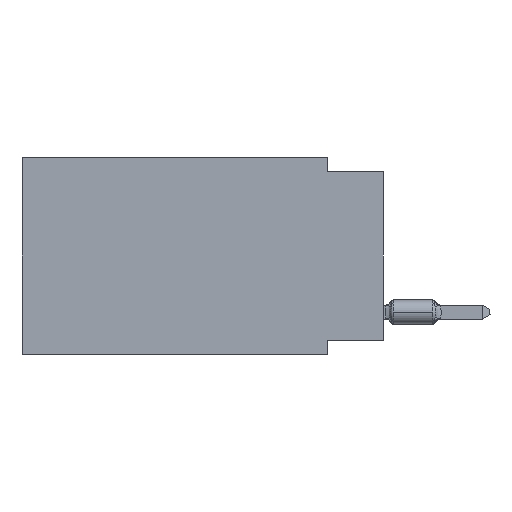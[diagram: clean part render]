
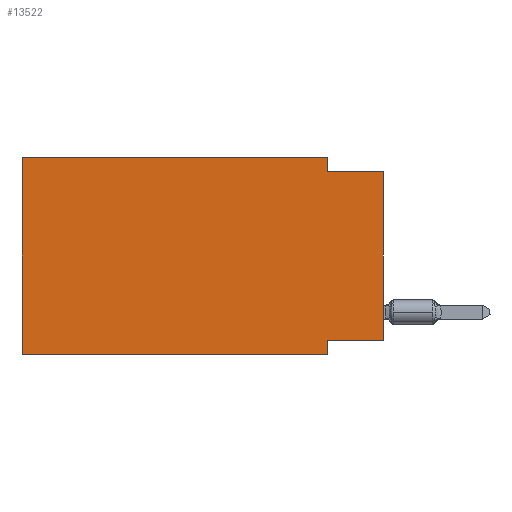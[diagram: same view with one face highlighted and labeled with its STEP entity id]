
A CAD part, left-side view. The second image highlights one B-rep face of the part: STEP entity #13522.
In plain terms, the highlighted planar face has unit normal (-1, 0, 0).
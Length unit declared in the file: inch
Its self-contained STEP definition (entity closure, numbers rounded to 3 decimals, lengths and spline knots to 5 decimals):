
#538 = DIRECTION ( 'NONE',  ( 0., -1., 0. ) ) ;
#586 = AXIS2_PLACEMENT_3D ( 'NONE', #4851, #16879, #795 ) ;
#795 = DIRECTION ( 'NONE',  ( 0., 0., -1. ) ) ;
#1550 = LINE ( 'NONE', #17487, #2868 ) ;
#1710 = EDGE_CURVE ( 'NONE', #11236, #19145, #3742, .T. ) ;
#1759 = VECTOR ( 'NONE', #21391, 39.37008 ) ;
#1805 = ORIENTED_EDGE ( 'NONE', *, *, #22641, .F. ) ;
#1933 = CARTESIAN_POINT ( 'NONE',  ( 0., 0.645, 0. ) ) ;
#2117 = LINE ( 'NONE', #16109, #18121 ) ;
#2248 = LINE ( 'NONE', #5902, #17907 ) ;
#2738 = VERTEX_POINT ( 'NONE', #16728 ) ;
#2868 = VECTOR ( 'NONE', #13320, 39.37008 ) ;
#2891 = FACE_OUTER_BOUND ( 'NONE', #11334, .T. ) ;
#3742 = LINE ( 'NONE', #13814, #11205 ) ;
#4851 = CARTESIAN_POINT ( 'NONE',  ( 0., 0.645, 0. ) ) ;
#5180 = VECTOR ( 'NONE', #25358, 39.37008 ) ;
#5387 = ORIENTED_EDGE ( 'NONE', *, *, #1710, .F. ) ;
#5389 = CARTESIAN_POINT ( 'NONE',  ( 0., 0.645, 0. ) ) ;
#5573 = ORIENTED_EDGE ( 'NONE', *, *, #20639, .F. ) ;
#5746 = LINE ( 'NONE', #17381, #5180 ) ;
#5902 = CARTESIAN_POINT ( 'NONE',  ( 0., 0.645, 0. ) ) ;
#7268 = CARTESIAN_POINT ( 'NONE',  ( 0., 0., -0.325 ) ) ;
#9048 = VERTEX_POINT ( 'NONE', #7268 ) ;
#10136 = VERTEX_POINT ( 'NONE', #16590 ) ;
#10343 = DIRECTION ( 'NONE',  ( 0., 1., 0. ) ) ;
#10454 = VERTEX_POINT ( 'NONE', #1933 ) ;
#11205 = VECTOR ( 'NONE', #11857, 39.37008 ) ;
#11236 = VERTEX_POINT ( 'NONE', #13699 ) ;
#11334 = EDGE_LOOP ( 'NONE', ( #23198, #21685, #5387, #5573, #18669, #18942, #20946, #1805 ) ) ;
#11542 = DIRECTION ( 'NONE',  ( 0., 0., 1. ) ) ;
#11857 = DIRECTION ( 'NONE',  ( 0., 0., -1. ) ) ;
#12547 = LINE ( 'NONE', #16211, #22579 ) ;
#12729 = CARTESIAN_POINT ( 'NONE',  ( 0., 0.1, -0.025 ) ) ;
#13320 = DIRECTION ( 'NONE',  ( 0., -1., 0. ) ) ;
#13522 = ADVANCED_FACE ( 'NONE', ( #2891 ), #20536, .F. ) ;
#13563 = LINE ( 'NONE', #17591, #1759 ) ;
#13699 = CARTESIAN_POINT ( 'NONE',  ( 0., 0.1, 0. ) ) ;
#13814 = CARTESIAN_POINT ( 'NONE',  ( 0., 0.1, 0. ) ) ;
#13923 = EDGE_CURVE ( 'NONE', #9048, #15624, #12547, .T. ) ;
#15539 = EDGE_CURVE ( 'NONE', #19145, #15624, #13563, .T. ) ;
#15624 = VERTEX_POINT ( 'NONE', #21522 ) ;
#16109 = CARTESIAN_POINT ( 'NONE',  ( 0., 0., -0.325 ) ) ;
#16211 = CARTESIAN_POINT ( 'NONE',  ( 0., 0., 0. ) ) ;
#16590 = CARTESIAN_POINT ( 'NONE',  ( 0., 0.1, -0.325 ) ) ;
#16728 = CARTESIAN_POINT ( 'NONE',  ( 0., 0.645, -0.35 ) ) ;
#16879 = DIRECTION ( 'NONE',  ( 1., 0., 0. ) ) ;
#17381 = CARTESIAN_POINT ( 'NONE',  ( 0., 0.1, -0.35 ) ) ;
#17487 = CARTESIAN_POINT ( 'NONE',  ( 0., 0.645, -0.35 ) ) ;
#17591 = CARTESIAN_POINT ( 'NONE',  ( 0., 0., -0.025 ) ) ;
#17907 = VECTOR ( 'NONE', #538, 39.37008 ) ;
#18121 = VECTOR ( 'NONE', #10343, 39.37008 ) ;
#18153 = VERTEX_POINT ( 'NONE', #23877 ) ;
#18669 = ORIENTED_EDGE ( 'NONE', *, *, #20499, .F. ) ;
#18942 = ORIENTED_EDGE ( 'NONE', *, *, #25553, .T. ) ;
#19145 = VERTEX_POINT ( 'NONE', #12729 ) ;
#20499 = EDGE_CURVE ( 'NONE', #2738, #10454, #23694, .T. ) ;
#20504 = DIRECTION ( 'NONE',  ( 0., 0., 1. ) ) ;
#20536 = PLANE ( 'NONE',  #586 ) ;
#20639 = EDGE_CURVE ( 'NONE', #10454, #11236, #2248, .T. ) ;
#20946 = ORIENTED_EDGE ( 'NONE', *, *, #22895, .F. ) ;
#21391 = DIRECTION ( 'NONE',  ( 0., -1., 0. ) ) ;
#21522 = CARTESIAN_POINT ( 'NONE',  ( 0., 0., -0.025 ) ) ;
#21679 = VECTOR ( 'NONE', #11542, 39.37008 ) ;
#21685 = ORIENTED_EDGE ( 'NONE', *, *, #15539, .F. ) ;
#22579 = VECTOR ( 'NONE', #20504, 39.37008 ) ;
#22641 = EDGE_CURVE ( 'NONE', #9048, #10136, #2117, .T. ) ;
#22895 = EDGE_CURVE ( 'NONE', #10136, #18153, #5746, .T. ) ;
#23198 = ORIENTED_EDGE ( 'NONE', *, *, #13923, .T. ) ;
#23694 = LINE ( 'NONE', #5389, #21679 ) ;
#23877 = CARTESIAN_POINT ( 'NONE',  ( 0., 0.1, -0.35 ) ) ;
#25358 = DIRECTION ( 'NONE',  ( 0., 0., -1. ) ) ;
#25553 = EDGE_CURVE ( 'NONE', #2738, #18153, #1550, .T. ) ;
